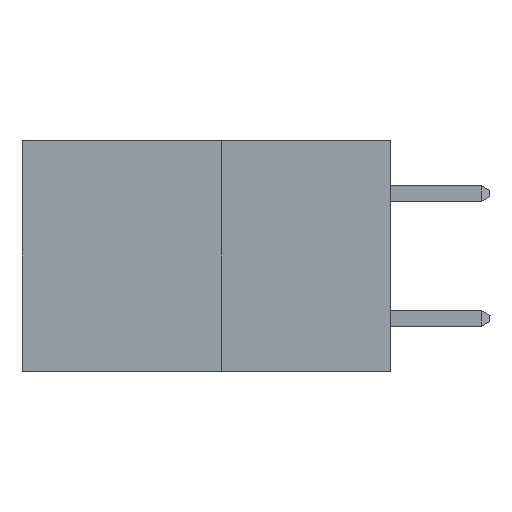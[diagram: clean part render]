
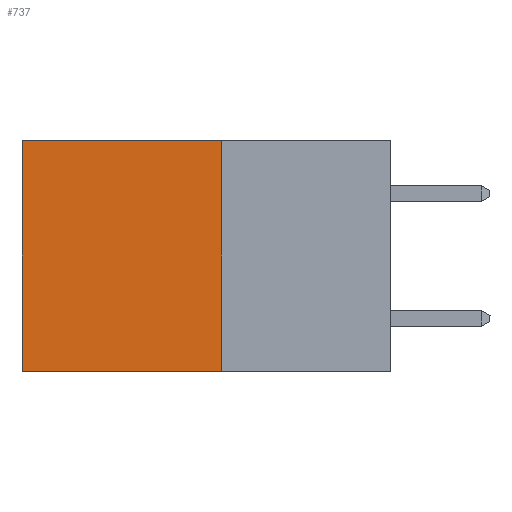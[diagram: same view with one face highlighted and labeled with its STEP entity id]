
A CAD part, left-side view. The second image highlights one B-rep face of the part: STEP entity #737.
In plain terms, the highlighted planar face has unit normal (-1, 0, 0).
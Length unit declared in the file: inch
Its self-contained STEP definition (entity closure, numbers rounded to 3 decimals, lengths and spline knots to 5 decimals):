
#737 = ADVANCED_FACE ( 'NONE', ( #2455 ), #9738, .F. ) ;
#1106 = CARTESIAN_POINT ( 'NONE',  ( 0.277, 0.59, -0.37 ) ) ;
#1500 = VECTOR ( 'NONE', #9111, 39.37008 ) ;
#1618 = LINE ( 'NONE', #10068, #7819 ) ;
#1805 = LINE ( 'NONE', #7503, #1500 ) ;
#1884 = DIRECTION ( 'NONE',  ( 0., 0., -1. ) ) ;
#2310 = VECTOR ( 'NONE', #1884, 39.37008 ) ;
#2455 = FACE_OUTER_BOUND ( 'NONE', #2475, .T. ) ;
#2475 = EDGE_LOOP ( 'NONE', ( #7621, #5153, #5121, #5391 ) ) ;
#3123 = EDGE_CURVE ( 'NONE', #3127, #8789, #1618, .T. ) ;
#3127 = VERTEX_POINT ( 'NONE', #6221 ) ;
#3166 = AXIS2_PLACEMENT_3D ( 'NONE', #9604, #9240, #3638 ) ;
#3638 = DIRECTION ( 'NONE',  ( 0., 0., -1. ) ) ;
#4374 = EDGE_CURVE ( 'NONE', #7484, #5294, #6657, .T. ) ;
#4803 = EDGE_CURVE ( 'NONE', #8789, #5294, #7153, .T. ) ;
#4918 = EDGE_CURVE ( 'NONE', #3127, #7484, #1805, .T. ) ;
#4963 = VECTOR ( 'NONE', #8881, 39.37008 ) ;
#5121 = ORIENTED_EDGE ( 'NONE', *, *, #3123, .F. ) ;
#5153 = ORIENTED_EDGE ( 'NONE', *, *, #4803, .F. ) ;
#5294 = VERTEX_POINT ( 'NONE', #9511 ) ;
#5391 = ORIENTED_EDGE ( 'NONE', *, *, #4918, .T. ) ;
#5505 = CARTESIAN_POINT ( 'NONE',  ( 0.277, 0.59, 0. ) ) ;
#6221 = CARTESIAN_POINT ( 'NONE',  ( 0.277, 0.27, 0. ) ) ;
#6286 = DIRECTION ( 'NONE',  ( 0., 0., -1. ) ) ;
#6657 = LINE ( 'NONE', #1106, #2310 ) ;
#7153 = LINE ( 'NONE', #8844, #4963 ) ;
#7484 = VERTEX_POINT ( 'NONE', #5505 ) ;
#7503 = CARTESIAN_POINT ( 'NONE',  ( 0.277, 0.27, 0. ) ) ;
#7621 = ORIENTED_EDGE ( 'NONE', *, *, #4374, .T. ) ;
#7819 = VECTOR ( 'NONE', #6286, 39.37008 ) ;
#8734 = CARTESIAN_POINT ( 'NONE',  ( 0.277, 0.27, -0.37 ) ) ;
#8789 = VERTEX_POINT ( 'NONE', #8734 ) ;
#8844 = CARTESIAN_POINT ( 'NONE',  ( 0.277, 0.27, -0.37 ) ) ;
#8881 = DIRECTION ( 'NONE',  ( 0., 1., 0. ) ) ;
#9111 = DIRECTION ( 'NONE',  ( 0., 1., 0. ) ) ;
#9240 = DIRECTION ( 'NONE',  ( 1., 0., 0. ) ) ;
#9511 = CARTESIAN_POINT ( 'NONE',  ( 0.277, 0.59, -0.37 ) ) ;
#9604 = CARTESIAN_POINT ( 'NONE',  ( 0.277, 0.27, -0.37 ) ) ;
#9738 = PLANE ( 'NONE',  #3166 ) ;
#10068 = CARTESIAN_POINT ( 'NONE',  ( 0.277, 0.27, -0.37 ) ) ;
